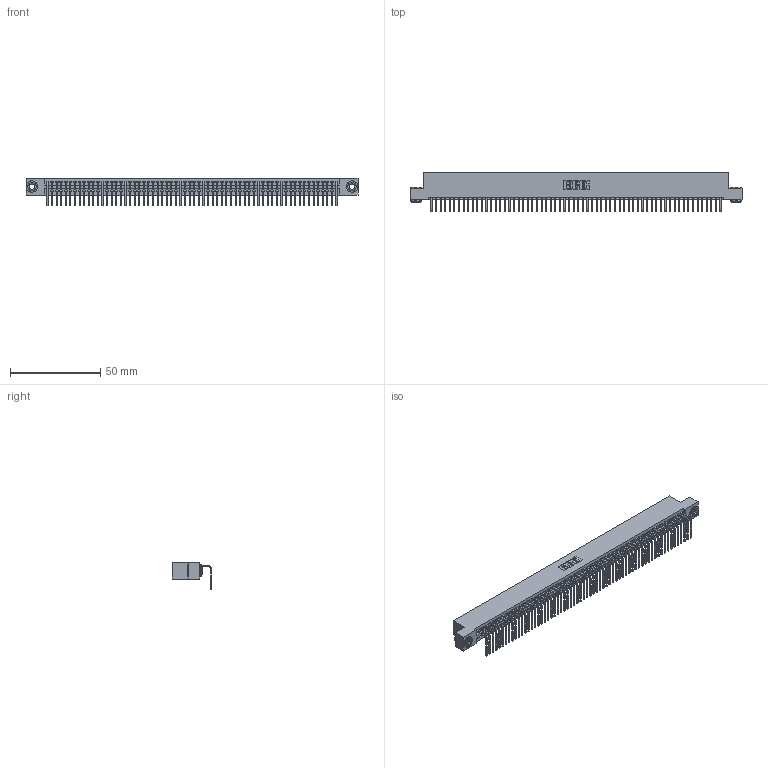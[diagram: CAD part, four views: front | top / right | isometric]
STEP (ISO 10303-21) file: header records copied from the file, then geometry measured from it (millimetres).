
FILE_DESCRIPTION (( 'STEP AP203' ), '1' );
FILE_NAME ('345-064-558-103.STEP', '2019-10-10T21:50:06', ( '' ), ( '' ), 'SwSTEP 2.0', 'SolidWorks 2016', '' );
FILE_SCHEMA (( 'CONFIG_CONTROL_DESIGN' ));
Length unit declared in the file: inch
Products named in the file (4): 345-292-001_558 Tail - 2; 345-250-002_345-250-002-102; 345-064-558-103; 345 Part_Flush Mounting Lugs - 0.156 Dia-TH
Assembly tree (67 placements, depth 2):
  345-064-558-103
    345 Part_Flush Mounting Lugs - 0.156 Dia-TH
    345-292-001_558 Tail - 2  x64
    345-250-002_345-250-002-102  x2
Bounding box: 183.77 x 21.83 x 15.37 mm (x, y, z)
Volume: 17867.4 mm3; surface area: 25510.6 mm2
Topology: 67 solids, 67 shells, 4004 faces, 12065 edges, 7954 vertices
Faces by surface type: plane 2778, cylinder 1218, cone 8
Entity records: 45940 total; most frequent: CARTESIAN_POINT 7935, ORIENTED_EDGE 7926, DIRECTION 6929, EDGE_CURVE 3963, LINE 3551, VECTOR 3551, VERTEX_POINT 2638, AXIS2_PLACEMENT_3D 1689
